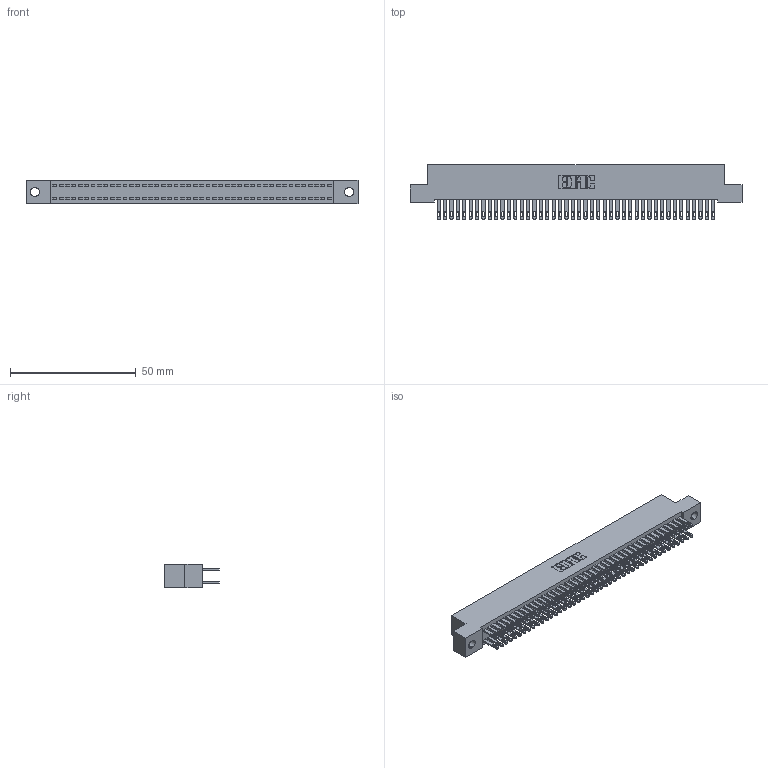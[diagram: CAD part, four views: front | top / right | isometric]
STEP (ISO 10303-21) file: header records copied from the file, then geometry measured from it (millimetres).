
FILE_DESCRIPTION (( 'STEP AP203' ), '1' );
FILE_NAME ('892-088-500-202.STEP', '2020-09-21T20:36:28', ( '' ), ( '' ), 'SwSTEP 2.0', 'SolidWorks 2020', '' );
FILE_SCHEMA (( 'CONFIG_CONTROL_DESIGN' ));
Length unit declared in the file: inch
Products named in the file (3): 842 Part_.128 Slot; 892-088-500-202; 345-292-001_345-293-100
Assembly tree (89 placements, depth 2):
  892-088-500-202
    842 Part_.128 Slot
    345-292-001_345-293-100  x88
Bounding box: 132.08 x 21.85 x 9.4 mm (x, y, z)
Volume: 12093.6 mm3; surface area: 20336.7 mm2
Topology: 89 solids, 89 shells, 4338 faces, 13247 edges, 8830 vertices
Faces by surface type: plane 2710, cylinder 1628
Entity records: 27981 total; most frequent: CARTESIAN_POINT 4634, ORIENTED_EDGE 4570, DIRECTION 3957, EDGE_CURVE 2285, VECTOR 2153, LINE 2153, VERTEX_POINT 1522, AXIS2_PLACEMENT_3D 902
